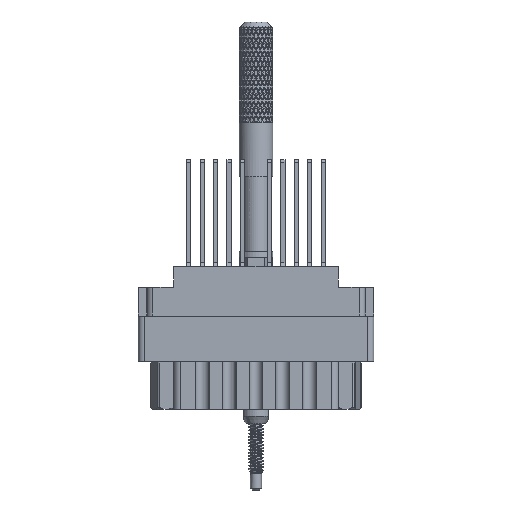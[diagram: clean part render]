
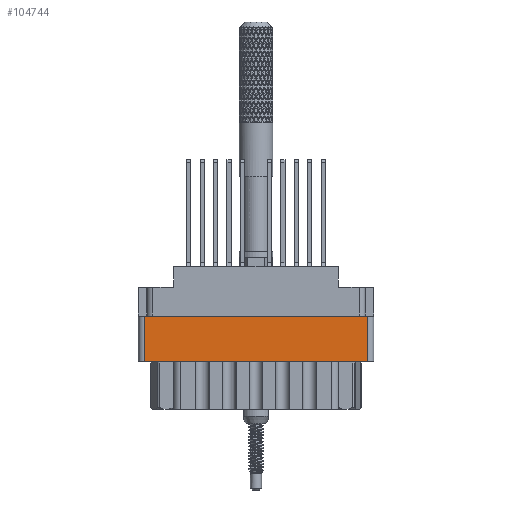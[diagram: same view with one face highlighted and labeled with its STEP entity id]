
A CAD part, front view. The second image highlights one B-rep face of the part: STEP entity #104744.
In plain terms, the highlighted planar face has unit normal (0, -1, 0).
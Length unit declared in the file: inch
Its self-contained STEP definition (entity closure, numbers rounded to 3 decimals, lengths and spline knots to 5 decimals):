
#1133 = EDGE_LOOP ( 'NONE', ( #157084, #132301, #20008, #55258 ) ) ;
#1840 = PLANE ( 'NONE',  #172813 ) ;
#12410 = LINE ( 'NONE', #89230, #43138 ) ;
#17567 = VERTEX_POINT ( 'NONE', #185370 ) ;
#20008 = ORIENTED_EDGE ( 'NONE', *, *, #53781, .F. ) ;
#30723 = VERTEX_POINT ( 'NONE', #73965 ) ;
#30818 = VECTOR ( 'NONE', #72528, 39.37008 ) ;
#43138 = VECTOR ( 'NONE', #165649, 39.37008 ) ;
#44267 = DIRECTION ( 'NONE',  ( 0., -1., 0. ) ) ;
#53386 = LINE ( 'NONE', #142922, #67612 ) ;
#53781 = EDGE_CURVE ( 'NONE', #17567, #30723, #12410, .T. ) ;
#54572 = DIRECTION ( 'NONE',  ( 1., 0., 0. ) ) ;
#55258 = ORIENTED_EDGE ( 'NONE', *, *, #85123, .T. ) ;
#57976 = CARTESIAN_POINT ( 'NONE',  ( -0.624, -0.343, -0.798 ) ) ;
#67612 = VECTOR ( 'NONE', #54572, 39.37008 ) ;
#72528 = DIRECTION ( 'NONE',  ( 0., 0., -1. ) ) ;
#73965 = CARTESIAN_POINT ( 'NONE',  ( -0.624, -0.343, -0.529 ) ) ;
#74316 = LINE ( 'NONE', #118234, #131343 ) ;
#77628 = FACE_OUTER_BOUND ( 'NONE', #1133, .T. ) ;
#81682 = CARTESIAN_POINT ( 'NONE',  ( 0.624, -0.343, -0.277 ) ) ;
#82952 = LINE ( 'NONE', #57976, #30818 ) ;
#85123 = EDGE_CURVE ( 'NONE', #17567, #142724, #74316, .T. ) ;
#89230 = CARTESIAN_POINT ( 'NONE',  ( 0., -0.343, -0.529 ) ) ;
#104744 = ADVANCED_FACE ( 'NONE', ( #77628 ), #1840, .T. ) ;
#105949 = DIRECTION ( 'NONE',  ( 0., 0., -1. ) ) ;
#107932 = CARTESIAN_POINT ( 'NONE',  ( -0.656, -0.343, -0.798 ) ) ;
#118234 = CARTESIAN_POINT ( 'NONE',  ( 0.624, -0.343, -0.798 ) ) ;
#131343 = VECTOR ( 'NONE', #138143, 39.37008 ) ;
#132301 = ORIENTED_EDGE ( 'NONE', *, *, #142381, .T. ) ;
#138143 = DIRECTION ( 'NONE',  ( 0., 0., 1. ) ) ;
#142381 = EDGE_CURVE ( 'NONE', #161700, #30723, #82952, .T. ) ;
#142724 = VERTEX_POINT ( 'NONE', #81682 ) ;
#142922 = CARTESIAN_POINT ( 'NONE',  ( 0., -0.343, -0.277 ) ) ;
#157084 = ORIENTED_EDGE ( 'NONE', *, *, #158709, .F. ) ;
#158709 = EDGE_CURVE ( 'NONE', #161700, #142724, #53386, .T. ) ;
#161700 = VERTEX_POINT ( 'NONE', #194562 ) ;
#165649 = DIRECTION ( 'NONE',  ( -1., 0., 0. ) ) ;
#172813 = AXIS2_PLACEMENT_3D ( 'NONE', #107932, #44267, #105949 ) ;
#185370 = CARTESIAN_POINT ( 'NONE',  ( 0.624, -0.343, -0.529 ) ) ;
#194562 = CARTESIAN_POINT ( 'NONE',  ( -0.624, -0.343, -0.277 ) ) ;
